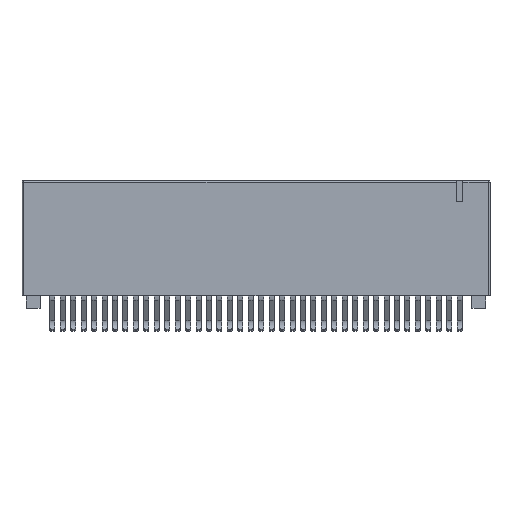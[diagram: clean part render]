
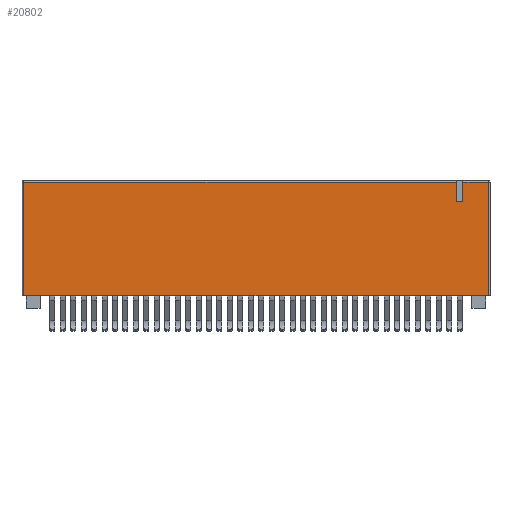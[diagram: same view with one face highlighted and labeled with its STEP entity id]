
A CAD part, top view. The second image highlights one B-rep face of the part: STEP entity #20802.
In plain terms, the highlighted planar face has unit normal (0, 0, 1).
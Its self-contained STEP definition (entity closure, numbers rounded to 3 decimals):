
#469 = EDGE_LOOP ( 'NONE', ( #13379, #27452, #27107, #11039, #27437, #1744, #5706, #19357 ) ) ;
#853 = DIRECTION ( 'NONE',  ( 0., 1., 0. ) ) ;
#1045 = FACE_OUTER_BOUND ( 'NONE', #469, .T. ) ;
#1328 = VERTEX_POINT ( 'NONE', #22133 ) ;
#1509 = DIRECTION ( 'NONE',  ( -1., 0., 0. ) ) ;
#1744 = ORIENTED_EDGE ( 'NONE', *, *, #8350, .T. ) ;
#1917 = DIRECTION ( 'NONE',  ( -1., 0., 0. ) ) ;
#2301 = VERTEX_POINT ( 'NONE', #7829 ) ;
#2724 = VECTOR ( 'NONE', #31004, 1000. ) ;
#3712 = VECTOR ( 'NONE', #6177, 1000. ) ;
#4352 = EDGE_CURVE ( 'NONE', #19608, #17273, #11323, .T. ) ;
#5533 = EDGE_CURVE ( 'NONE', #1328, #2301, #10600, .T. ) ;
#5706 = ORIENTED_EDGE ( 'NONE', *, *, #4352, .T. ) ;
#5712 = EDGE_CURVE ( 'NONE', #12309, #20050, #20826, .T. ) ;
#6022 = CARTESIAN_POINT ( 'NONE',  ( 52.825, 12.95, 0. ) ) ;
#6177 = DIRECTION ( 'NONE',  ( 1., 0., 0. ) ) ;
#6337 = CARTESIAN_POINT ( 'NONE',  ( 56.7, 15.3, 0. ) ) ;
#7829 = CARTESIAN_POINT ( 'NONE',  ( 0.2, 1.5, 0. ) ) ;
#8002 = CARTESIAN_POINT ( 'NONE',  ( 53.605, 15.3, 0. ) ) ;
#8350 = EDGE_CURVE ( 'NONE', #1328, #19608, #22746, .T. ) ;
#8421 = VECTOR ( 'NONE', #25202, 1000. ) ;
#8578 = CARTESIAN_POINT ( 'NONE',  ( 52.825, 12.95, 0. ) ) ;
#9654 = EDGE_CURVE ( 'NONE', #20050, #17273, #12661, .T. ) ;
#10509 = CARTESIAN_POINT ( 'NONE',  ( 52.825, 12.95, 0. ) ) ;
#10563 = EDGE_CURVE ( 'NONE', #12309, #13865, #27525, .T. ) ;
#10600 = LINE ( 'NONE', #17529, #30864 ) ;
#11039 = ORIENTED_EDGE ( 'NONE', *, *, #23548, .T. ) ;
#11323 = LINE ( 'NONE', #13694, #2724 ) ;
#12165 = VERTEX_POINT ( 'NONE', #29542 ) ;
#12309 = VERTEX_POINT ( 'NONE', #8578 ) ;
#12661 = LINE ( 'NONE', #17383, #12977 ) ;
#12977 = VECTOR ( 'NONE', #24803, 1000. ) ;
#13379 = ORIENTED_EDGE ( 'NONE', *, *, #5712, .F. ) ;
#13483 = PLANE ( 'NONE',  #20962 ) ;
#13694 = CARTESIAN_POINT ( 'NONE',  ( 0., 15.3, 0. ) ) ;
#13865 = VERTEX_POINT ( 'NONE', #30590 ) ;
#14321 = CARTESIAN_POINT ( 'NONE',  ( 53.605, 12.95, 0. ) ) ;
#15320 = DIRECTION ( 'NONE',  ( -1., 0., 0. ) ) ;
#17273 = VERTEX_POINT ( 'NONE', #8002 ) ;
#17383 = CARTESIAN_POINT ( 'NONE',  ( 53.605, 12.95, 0. ) ) ;
#17529 = CARTESIAN_POINT ( 'NONE',  ( 56.9, 1.5, 0. ) ) ;
#18100 = LINE ( 'NONE', #24882, #8421 ) ;
#18760 = LINE ( 'NONE', #30589, #30111 ) ;
#19357 = ORIENTED_EDGE ( 'NONE', *, *, #9654, .F. ) ;
#19535 = VECTOR ( 'NONE', #29727, 1000. ) ;
#19608 = VERTEX_POINT ( 'NONE', #6337 ) ;
#20050 = VERTEX_POINT ( 'NONE', #14321 ) ;
#20729 = DIRECTION ( 'NONE',  ( 0., 0., -1. ) ) ;
#20802 = ADVANCED_FACE ( 'NONE', ( #1045 ), #13483, .F. ) ;
#20826 = LINE ( 'NONE', #6022, #3712 ) ;
#20880 = CARTESIAN_POINT ( 'NONE',  ( 0., 15.5, 0. ) ) ;
#20962 = AXIS2_PLACEMENT_3D ( 'NONE', #20880, #20729, #1509 ) ;
#22133 = CARTESIAN_POINT ( 'NONE',  ( 56.7, 1.5, 0. ) ) ;
#22463 = VECTOR ( 'NONE', #853, 1000. ) ;
#22746 = LINE ( 'NONE', #27320, #22463 ) ;
#23548 = EDGE_CURVE ( 'NONE', #12165, #2301, #18100, .T. ) ;
#24803 = DIRECTION ( 'NONE',  ( 0., 1., 0. ) ) ;
#24882 = CARTESIAN_POINT ( 'NONE',  ( 0.2, 15.5, 0. ) ) ;
#25202 = DIRECTION ( 'NONE',  ( 0., -1., 0. ) ) ;
#26690 = EDGE_CURVE ( 'NONE', #13865, #12165, #18760, .T. ) ;
#27107 = ORIENTED_EDGE ( 'NONE', *, *, #26690, .T. ) ;
#27320 = CARTESIAN_POINT ( 'NONE',  ( 56.7, 15.5, 0. ) ) ;
#27437 = ORIENTED_EDGE ( 'NONE', *, *, #5533, .F. ) ;
#27452 = ORIENTED_EDGE ( 'NONE', *, *, #10563, .T. ) ;
#27525 = LINE ( 'NONE', #10509, #19535 ) ;
#29542 = CARTESIAN_POINT ( 'NONE',  ( 0.2, 15.3, 0. ) ) ;
#29727 = DIRECTION ( 'NONE',  ( 0., 1., 0. ) ) ;
#30111 = VECTOR ( 'NONE', #1917, 1000. ) ;
#30589 = CARTESIAN_POINT ( 'NONE',  ( 0., 15.3, 0. ) ) ;
#30590 = CARTESIAN_POINT ( 'NONE',  ( 52.825, 15.3, 0. ) ) ;
#30864 = VECTOR ( 'NONE', #15320, 1000. ) ;
#31004 = DIRECTION ( 'NONE',  ( -1., 0., 0. ) ) ;
